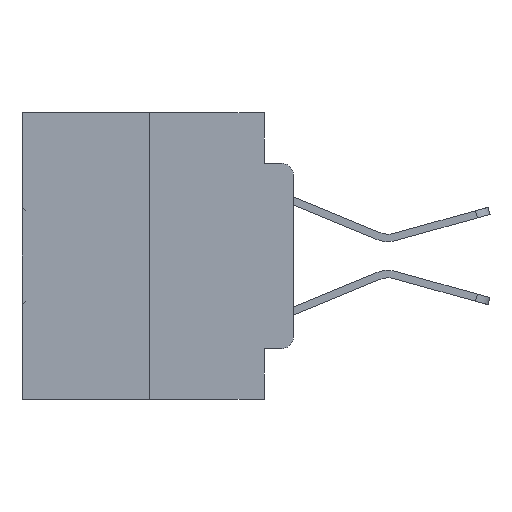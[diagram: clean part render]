
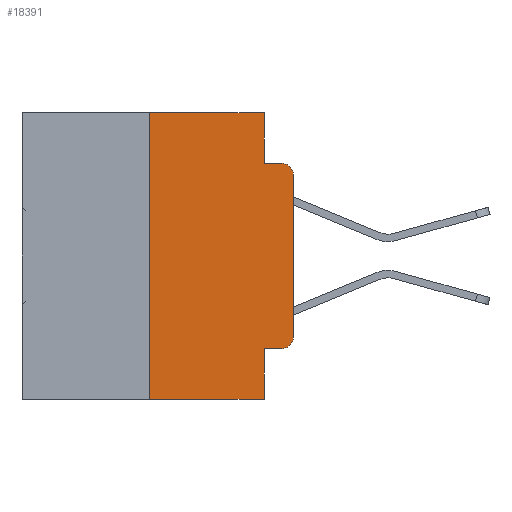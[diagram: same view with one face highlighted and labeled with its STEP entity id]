
A CAD part, left-side view. The second image highlights one B-rep face of the part: STEP entity #18391.
In plain terms, the highlighted planar face has unit normal (-1, 0, 0).
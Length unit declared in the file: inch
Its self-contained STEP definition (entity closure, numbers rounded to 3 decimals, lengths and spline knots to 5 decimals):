
#100 = DIRECTION ( 'NONE',  ( 0., -1., 0. ) ) ;
#223 = CARTESIAN_POINT ( 'NONE',  ( 0., 0., 0. ) ) ;
#1543 = VECTOR ( 'NONE', #100, 39.37008 ) ;
#1551 = ORIENTED_EDGE ( 'NONE', *, *, #21856, .T. ) ;
#2871 = VERTEX_POINT ( 'NONE', #15138 ) ;
#3213 = VERTEX_POINT ( 'NONE', #3848 ) ;
#3507 = VERTEX_POINT ( 'NONE', #8728 ) ;
#3848 = CARTESIAN_POINT ( 'NONE',  ( 0., 0., -0.3915 ) ) ;
#4082 = DIRECTION ( 'NONE',  ( -1., 0., 0. ) ) ;
#4367 = VECTOR ( 'NONE', #23723, 39.37008 ) ;
#4521 = CIRCLE ( 'NONE', #28168, 0.02 ) ;
#4909 = VECTOR ( 'NONE', #31777, 39.37008 ) ;
#4921 = VECTOR ( 'NONE', #19386, 39.37008 ) ;
#5006 = VECTOR ( 'NONE', #13337, 39.37008 ) ;
#5401 = LINE ( 'NONE', #23897, #1543 ) ;
#5960 = EDGE_CURVE ( 'NONE', #23671, #3507, #16683, .T. ) ;
#6232 = EDGE_CURVE ( 'NONE', #3213, #29351, #32822, .T. ) ;
#6631 = PLANE ( 'NONE',  #18228 ) ;
#6777 = EDGE_CURVE ( 'NONE', #18717, #3213, #4521, .T. ) ;
#7245 = DIRECTION ( 'NONE',  ( 0., 0., -1. ) ) ;
#7711 = LINE ( 'NONE', #26720, #5006 ) ;
#7729 = ORIENTED_EDGE ( 'NONE', *, *, #6777, .T. ) ;
#7772 = CARTESIAN_POINT ( 'NONE',  ( 0., 0.02, -0.4115 ) ) ;
#8129 = VERTEX_POINT ( 'NONE', #25557 ) ;
#8147 = LINE ( 'NONE', #10629, #4909 ) ;
#8728 = CARTESIAN_POINT ( 'NONE',  ( 0., 0.051, -0.5 ) ) ;
#9531 = CARTESIAN_POINT ( 'NONE',  ( 0., 0.02, -0.0885 ) ) ;
#10629 = CARTESIAN_POINT ( 'NONE',  ( 0., 0.051, -0.0885 ) ) ;
#13337 = DIRECTION ( 'NONE',  ( 0., -1., 0. ) ) ;
#13726 = ORIENTED_EDGE ( 'NONE', *, *, #33449, .T. ) ;
#14511 = ORIENTED_EDGE ( 'NONE', *, *, #21343, .F. ) ;
#14568 = VERTEX_POINT ( 'NONE', #19538 ) ;
#14715 = CARTESIAN_POINT ( 'NONE',  ( 0., 0.051, -0.4115 ) ) ;
#15138 = CARTESIAN_POINT ( 'NONE',  ( 0., 0.051, -0.0885 ) ) ;
#15960 = ORIENTED_EDGE ( 'NONE', *, *, #21371, .F. ) ;
#16170 = VECTOR ( 'NONE', #32483, 39.37008 ) ;
#16683 = LINE ( 'NONE', #19315, #4921 ) ;
#17008 = EDGE_LOOP ( 'NONE', ( #30367, #13726, #17750, #26023, #15960, #14511, #1551, #28322, #33095, #7729 ) ) ;
#17528 = DIRECTION ( 'NONE',  ( 1., 0., 0. ) ) ;
#17750 = ORIENTED_EDGE ( 'NONE', *, *, #30844, .F. ) ;
#18228 = AXIS2_PLACEMENT_3D ( 'NONE', #20177, #17528, #33911 ) ;
#18391 = ADVANCED_FACE ( 'NONE', ( #34088 ), #6631, .F. ) ;
#18432 = VECTOR ( 'NONE', #30731, 39.37008 ) ;
#18602 = CARTESIAN_POINT ( 'NONE',  ( 0., 0.25, 0. ) ) ;
#18717 = VERTEX_POINT ( 'NONE', #7772 ) ;
#19315 = CARTESIAN_POINT ( 'NONE',  ( 0., 0.051, 0. ) ) ;
#19386 = DIRECTION ( 'NONE',  ( 0., 0., -1. ) ) ;
#19538 = CARTESIAN_POINT ( 'NONE',  ( 0., 0.051, 0. ) ) ;
#19855 = DIRECTION ( 'NONE',  ( -1., 0., 0. ) ) ;
#20130 = LINE ( 'NONE', #28600, #18432 ) ;
#20177 = CARTESIAN_POINT ( 'NONE',  ( 0., 0.473, 0. ) ) ;
#21343 = EDGE_CURVE ( 'NONE', #8129, #30110, #25678, .T. ) ;
#21371 = EDGE_CURVE ( 'NONE', #30110, #14568, #5401, .T. ) ;
#21856 = EDGE_CURVE ( 'NONE', #8129, #3507, #20130, .T. ) ;
#23671 = VERTEX_POINT ( 'NONE', #14715 ) ;
#23723 = DIRECTION ( 'NONE',  ( 0., 0., 1. ) ) ;
#23897 = CARTESIAN_POINT ( 'NONE',  ( 0., 0.473, 0. ) ) ;
#25233 = CIRCLE ( 'NONE', #33104, 0.02 ) ;
#25237 = VECTOR ( 'NONE', #31923, 39.37008 ) ;
#25557 = CARTESIAN_POINT ( 'NONE',  ( 0., 0.25, -0.5 ) ) ;
#25678 = LINE ( 'NONE', #18602, #4367 ) ;
#26023 = ORIENTED_EDGE ( 'NONE', *, *, #31748, .F. ) ;
#26720 = CARTESIAN_POINT ( 'NONE',  ( 0., 0.051, -0.4115 ) ) ;
#26949 = VERTEX_POINT ( 'NONE', #9531 ) ;
#27609 = CARTESIAN_POINT ( 'NONE',  ( 0., 0.25, 0. ) ) ;
#28099 = CARTESIAN_POINT ( 'NONE',  ( 0., 0., -0.1085 ) ) ;
#28168 = AXIS2_PLACEMENT_3D ( 'NONE', #30639, #19855, #30304 ) ;
#28322 = ORIENTED_EDGE ( 'NONE', *, *, #5960, .F. ) ;
#28565 = CARTESIAN_POINT ( 'NONE',  ( 0., 0.02, -0.1085 ) ) ;
#28600 = CARTESIAN_POINT ( 'NONE',  ( 0., 0.473, -0.5 ) ) ;
#29351 = VERTEX_POINT ( 'NONE', #28099 ) ;
#30110 = VERTEX_POINT ( 'NONE', #27609 ) ;
#30304 = DIRECTION ( 'NONE',  ( 0., 0., -1. ) ) ;
#30367 = ORIENTED_EDGE ( 'NONE', *, *, #6232, .T. ) ;
#30639 = CARTESIAN_POINT ( 'NONE',  ( 0., 0.02, -0.3915 ) ) ;
#30731 = DIRECTION ( 'NONE',  ( 0., -1., 0. ) ) ;
#30844 = EDGE_CURVE ( 'NONE', #2871, #26949, #8147, .T. ) ;
#31748 = EDGE_CURVE ( 'NONE', #14568, #2871, #32101, .T. ) ;
#31777 = DIRECTION ( 'NONE',  ( 0., -1., 0. ) ) ;
#31923 = DIRECTION ( 'NONE',  ( 0., 0., -1. ) ) ;
#32101 = LINE ( 'NONE', #32263, #25237 ) ;
#32263 = CARTESIAN_POINT ( 'NONE',  ( 0., 0.051, 0. ) ) ;
#32483 = DIRECTION ( 'NONE',  ( 0., 0., 1. ) ) ;
#32822 = LINE ( 'NONE', #223, #16170 ) ;
#33095 = ORIENTED_EDGE ( 'NONE', *, *, #34007, .T. ) ;
#33104 = AXIS2_PLACEMENT_3D ( 'NONE', #28565, #4082, #7245 ) ;
#33449 = EDGE_CURVE ( 'NONE', #29351, #26949, #25233, .T. ) ;
#33911 = DIRECTION ( 'NONE',  ( 0., 0., -1. ) ) ;
#34007 = EDGE_CURVE ( 'NONE', #23671, #18717, #7711, .T. ) ;
#34088 = FACE_OUTER_BOUND ( 'NONE', #17008, .T. ) ;
